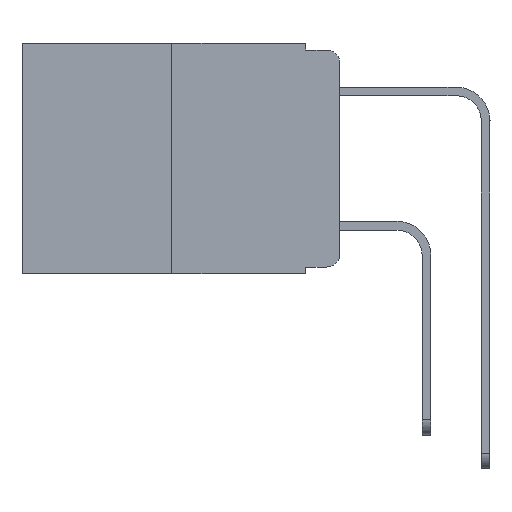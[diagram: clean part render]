
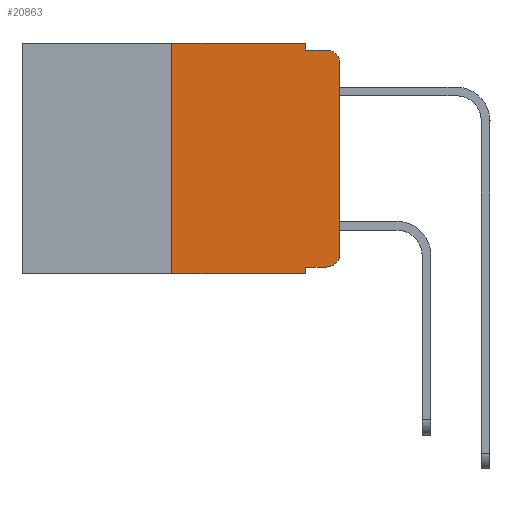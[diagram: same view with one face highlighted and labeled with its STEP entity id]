
A CAD part, left-side view. The second image highlights one B-rep face of the part: STEP entity #20863.
In plain terms, the highlighted planar face has unit normal (-1, 0, 0).
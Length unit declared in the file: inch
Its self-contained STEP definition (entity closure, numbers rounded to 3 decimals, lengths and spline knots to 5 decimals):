
#27 = DIRECTION ( 'NONE',  ( 0., -1., 0. ) ) ;
#798 = FACE_OUTER_BOUND ( 'NONE', #19861, .T. ) ;
#1643 = ORIENTED_EDGE ( 'NONE', *, *, #20054, .F. ) ;
#1957 = VECTOR ( 'NONE', #9832, 39.37008 ) ;
#2775 = CARTESIAN_POINT ( 'NONE',  ( 0., 0., -0.313 ) ) ;
#2919 = CARTESIAN_POINT ( 'NONE',  ( 0., 0.25, 0. ) ) ;
#2991 = VERTEX_POINT ( 'NONE', #18607 ) ;
#3187 = LINE ( 'NONE', #25742, #19353 ) ;
#3204 = DIRECTION ( 'NONE',  ( 0., -1., 0. ) ) ;
#3206 = DIRECTION ( 'NONE',  ( 0., 0., -1. ) ) ;
#3499 = VECTOR ( 'NONE', #4408, 39.37008 ) ;
#4361 = VERTEX_POINT ( 'NONE', #2775 ) ;
#4408 = DIRECTION ( 'NONE',  ( 0., 0., 1. ) ) ;
#5282 = CARTESIAN_POINT ( 'NONE',  ( 0., 0.051, -0.01 ) ) ;
#5741 = CARTESIAN_POINT ( 'NONE',  ( 0., 0.02, -0.03 ) ) ;
#6231 = CARTESIAN_POINT ( 'NONE',  ( 0., 0.473, 0. ) ) ;
#6309 = DIRECTION ( 'NONE',  ( 1., 0., 0. ) ) ;
#6480 = CARTESIAN_POINT ( 'NONE',  ( 0., 0.25, 0. ) ) ;
#6939 = VERTEX_POINT ( 'NONE', #2919 ) ;
#6940 = EDGE_CURVE ( 'NONE', #2991, #4361, #14334, .T. ) ;
#7055 = CARTESIAN_POINT ( 'NONE',  ( 0., 0.02, -0.313 ) ) ;
#7473 = LINE ( 'NONE', #7823, #1957 ) ;
#7812 = DIRECTION ( 'NONE',  ( 0., 0., -1. ) ) ;
#7823 = CARTESIAN_POINT ( 'NONE',  ( 0., 0.051, -0.333 ) ) ;
#8423 = ORIENTED_EDGE ( 'NONE', *, *, #22386, .T. ) ;
#8665 = VERTEX_POINT ( 'NONE', #22923 ) ;
#8951 = CARTESIAN_POINT ( 'NONE',  ( 0., 0.051, 0. ) ) ;
#9019 = CARTESIAN_POINT ( 'NONE',  ( 0., 0.051, -0.333 ) ) ;
#9088 = DIRECTION ( 'NONE',  ( 0., 0., -1. ) ) ;
#9358 = ORIENTED_EDGE ( 'NONE', *, *, #25464, .F. ) ;
#9832 = DIRECTION ( 'NONE',  ( 0., -1., 0. ) ) ;
#9884 = VECTOR ( 'NONE', #3204, 39.37008 ) ;
#10192 = VECTOR ( 'NONE', #24879, 39.37008 ) ;
#10507 = LINE ( 'NONE', #5282, #9884 ) ;
#10759 = CARTESIAN_POINT ( 'NONE',  ( 0., 0.25, -0.343 ) ) ;
#10978 = VERTEX_POINT ( 'NONE', #10759 ) ;
#11342 = AXIS2_PLACEMENT_3D ( 'NONE', #6231, #6309, #20392 ) ;
#12307 = PLANE ( 'NONE',  #11342 ) ;
#12496 = CARTESIAN_POINT ( 'NONE',  ( 0., 0., 0. ) ) ;
#13205 = VERTEX_POINT ( 'NONE', #17661 ) ;
#13417 = VECTOR ( 'NONE', #27, 39.37008 ) ;
#13447 = ORIENTED_EDGE ( 'NONE', *, *, #6940, .T. ) ;
#13615 = VERTEX_POINT ( 'NONE', #23138 ) ;
#14138 = EDGE_CURVE ( 'NONE', #18410, #2991, #7473, .T. ) ;
#14268 = LINE ( 'NONE', #6480, #3499 ) ;
#14294 = VECTOR ( 'NONE', #22439, 39.37008 ) ;
#14334 = CIRCLE ( 'NONE', #21043, 0.02 ) ;
#16163 = EDGE_CURVE ( 'NONE', #6939, #13615, #18791, .T. ) ;
#16828 = LINE ( 'NONE', #8951, #10192 ) ;
#16914 = ORIENTED_EDGE ( 'NONE', *, *, #14138, .T. ) ;
#17661 = CARTESIAN_POINT ( 'NONE',  ( 0., 0., -0.03 ) ) ;
#17897 = EDGE_CURVE ( 'NONE', #13615, #21019, #16828, .T. ) ;
#18353 = VERTEX_POINT ( 'NONE', #24701 ) ;
#18410 = VERTEX_POINT ( 'NONE', #9019 ) ;
#18607 = CARTESIAN_POINT ( 'NONE',  ( 0., 0.02, -0.333 ) ) ;
#18791 = LINE ( 'NONE', #22309, #13417 ) ;
#18974 = AXIS2_PLACEMENT_3D ( 'NONE', #5741, #19851, #7812 ) ;
#19353 = VECTOR ( 'NONE', #25661, 39.37008 ) ;
#19491 = VECTOR ( 'NONE', #3206, 39.37008 ) ;
#19851 = DIRECTION ( 'NONE',  ( -1., 0., 0. ) ) ;
#19861 = EDGE_LOOP ( 'NONE', ( #8423, #20362, #1643, #23721, #20041, #21275, #24013, #9358, #16914, #13447 ) ) ;
#20041 = ORIENTED_EDGE ( 'NONE', *, *, #16163, .F. ) ;
#20054 = EDGE_CURVE ( 'NONE', #21019, #18353, #10507, .T. ) ;
#20362 = ORIENTED_EDGE ( 'NONE', *, *, #21363, .T. ) ;
#20392 = DIRECTION ( 'NONE',  ( 0., 0., -1. ) ) ;
#20863 = ADVANCED_FACE ( 'NONE', ( #798 ), #12307, .F. ) ;
#21019 = VERTEX_POINT ( 'NONE', #24655 ) ;
#21043 = AXIS2_PLACEMENT_3D ( 'NONE', #7055, #21091, #9088 ) ;
#21091 = DIRECTION ( 'NONE',  ( -1., 0., 0. ) ) ;
#21275 = ORIENTED_EDGE ( 'NONE', *, *, #23495, .F. ) ;
#21363 = EDGE_CURVE ( 'NONE', #13205, #18353, #25067, .T. ) ;
#21372 = CARTESIAN_POINT ( 'NONE',  ( 0., 0.051, 0. ) ) ;
#22309 = CARTESIAN_POINT ( 'NONE',  ( 0., 0.473, 0. ) ) ;
#22386 = EDGE_CURVE ( 'NONE', #4361, #13205, #24847, .T. ) ;
#22439 = DIRECTION ( 'NONE',  ( 0., 0., 1. ) ) ;
#22923 = CARTESIAN_POINT ( 'NONE',  ( 0., 0.051, -0.343 ) ) ;
#23138 = CARTESIAN_POINT ( 'NONE',  ( 0., 0.051, 0. ) ) ;
#23303 = EDGE_CURVE ( 'NONE', #10978, #8665, #3187, .T. ) ;
#23495 = EDGE_CURVE ( 'NONE', #10978, #6939, #14268, .T. ) ;
#23721 = ORIENTED_EDGE ( 'NONE', *, *, #17897, .F. ) ;
#24013 = ORIENTED_EDGE ( 'NONE', *, *, #23303, .T. ) ;
#24655 = CARTESIAN_POINT ( 'NONE',  ( 0., 0.051, -0.01 ) ) ;
#24701 = CARTESIAN_POINT ( 'NONE',  ( 0., 0.02, -0.01 ) ) ;
#24847 = LINE ( 'NONE', #12496, #14294 ) ;
#24879 = DIRECTION ( 'NONE',  ( 0., 0., -1. ) ) ;
#25067 = CIRCLE ( 'NONE', #18974, 0.02 ) ;
#25281 = LINE ( 'NONE', #21372, #19491 ) ;
#25464 = EDGE_CURVE ( 'NONE', #18410, #8665, #25281, .T. ) ;
#25661 = DIRECTION ( 'NONE',  ( 0., -1., 0. ) ) ;
#25742 = CARTESIAN_POINT ( 'NONE',  ( 0., 0.473, -0.343 ) ) ;
